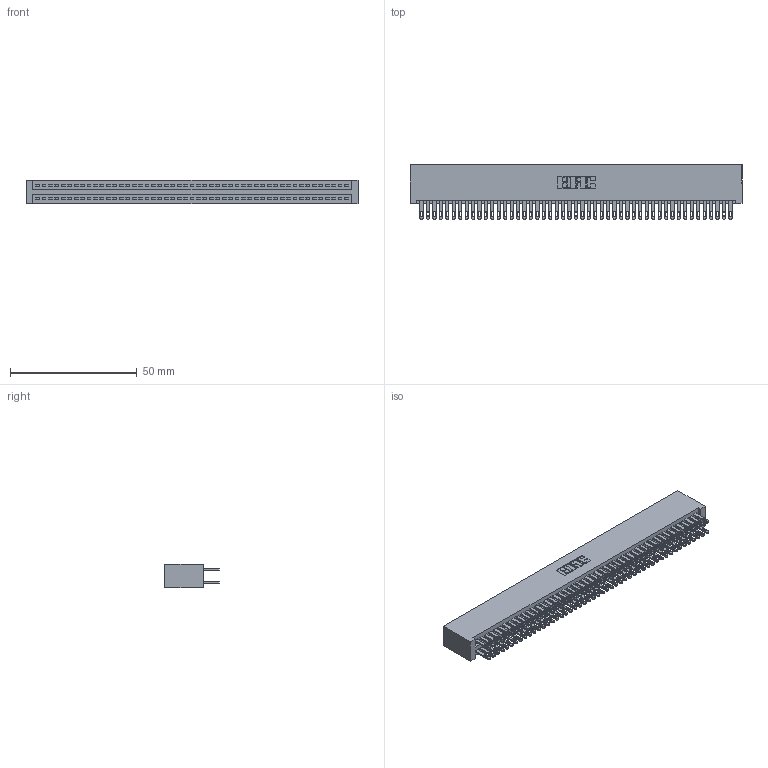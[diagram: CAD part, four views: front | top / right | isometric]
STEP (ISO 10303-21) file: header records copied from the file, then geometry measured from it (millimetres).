
FILE_DESCRIPTION (( 'STEP AP203' ), '1' );
FILE_NAME ('345-098-500-201.STEP', '2019-11-02T09:51:28', ( '' ), ( '' ), 'SwSTEP 2.0', 'SolidWorks 2016', '' );
FILE_SCHEMA (( 'CONFIG_CONTROL_DESIGN' ));
Length unit declared in the file: inch
Products named in the file (3): 345-098-500-201; 345-292-001_345-293-100; 345 Part_No Mounting Lugs
Assembly tree (99 placements, depth 2):
  345-098-500-201
    345 Part_No Mounting Lugs
    345-292-001_345-293-100  x98
Bounding box: 131.06 x 21.51 x 9.4 mm (x, y, z)
Volume: 13712 mm3; surface area: 21707.1 mm2
Topology: 99 solids, 99 shells, 4626 faces, 14135 edges, 9422 vertices
Faces by surface type: plane 2722, cylinder 1904
Entity records: 37157 total; most frequent: CARTESIAN_POINT 6220, ORIENTED_EDGE 6154, DIRECTION 5473, EDGE_CURVE 3077, VECTOR 2753, LINE 2753, VERTEX_POINT 2050, AXIS2_PLACEMENT_3D 1360
